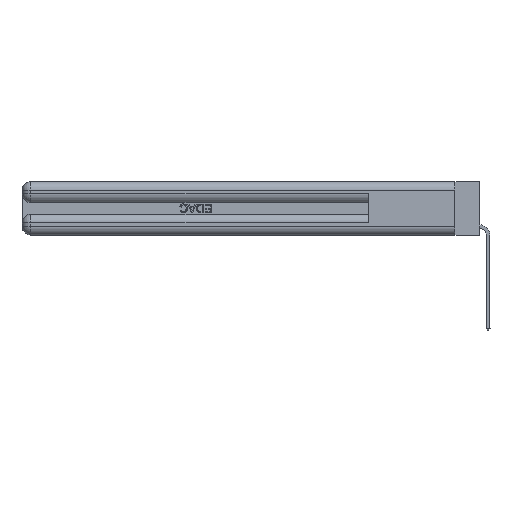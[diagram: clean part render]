
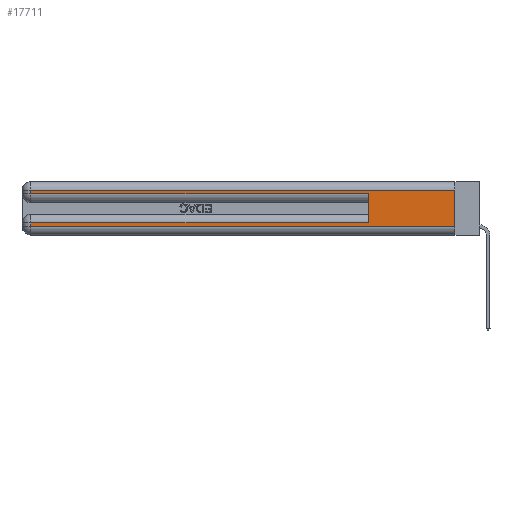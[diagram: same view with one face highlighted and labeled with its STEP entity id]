
A CAD part, left-side view. The second image highlights one B-rep face of the part: STEP entity #17711.
In plain terms, the highlighted planar face has unit normal (-1, 0, 0).
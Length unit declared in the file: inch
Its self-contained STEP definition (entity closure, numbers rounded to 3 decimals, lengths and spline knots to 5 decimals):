
#437 = CARTESIAN_POINT ( 'NONE',  ( 0., 0.6, 0.285 ) ) ;
#541 = AXIS2_PLACEMENT_3D ( 'NONE', #9061, #16422, #13409 ) ;
#1165 = VECTOR ( 'NONE', #8745, 39.37008 ) ;
#1166 = EDGE_CURVE ( 'NONE', #23944, #1646, #4770, .T. ) ;
#1267 = DIRECTION ( 'NONE',  ( 0., 0., -1. ) ) ;
#1416 = EDGE_CURVE ( 'NONE', #3021, #27083, #19693, .T. ) ;
#1646 = VERTEX_POINT ( 'NONE', #437 ) ;
#1948 = EDGE_CURVE ( 'NONE', #26313, #26884, #22142, .T. ) ;
#2638 = VECTOR ( 'NONE', #27305, 39.37008 ) ;
#3021 = VERTEX_POINT ( 'NONE', #27377 ) ;
#3228 = DIRECTION ( 'NONE',  ( 0., 0., -1. ) ) ;
#3637 = ORIENTED_EDGE ( 'NONE', *, *, #15374, .T. ) ;
#3994 = DIRECTION ( 'NONE',  ( 0., 1., 0. ) ) ;
#4770 = LINE ( 'NONE', #9004, #2638 ) ;
#4819 = LINE ( 'NONE', #27820, #1165 ) ;
#6630 = EDGE_CURVE ( 'NONE', #9397, #23944, #10506, .T. ) ;
#6666 = ORIENTED_EDGE ( 'NONE', *, *, #11618, .F. ) ;
#7908 = ORIENTED_EDGE ( 'NONE', *, *, #1948, .T. ) ;
#8669 = CARTESIAN_POINT ( 'NONE',  ( 0., 0., 0.31 ) ) ;
#8745 = DIRECTION ( 'NONE',  ( 0., 1., 0. ) ) ;
#8899 = ORIENTED_EDGE ( 'NONE', *, *, #1416, .F. ) ;
#9004 = CARTESIAN_POINT ( 'NONE',  ( 0., 0., 0.285 ) ) ;
#9061 = CARTESIAN_POINT ( 'NONE',  ( 0., 0., 0.37 ) ) ;
#9397 = VERTEX_POINT ( 'NONE', #14711 ) ;
#10204 = VECTOR ( 'NONE', #1267, 39.37008 ) ;
#10211 = CARTESIAN_POINT ( 'NONE',  ( 0., 2.94, 0.37 ) ) ;
#10324 = LINE ( 'NONE', #12427, #22272 ) ;
#10506 = LINE ( 'NONE', #10211, #10204 ) ;
#10920 = VECTOR ( 'NONE', #24571, 39.37008 ) ;
#11618 = EDGE_CURVE ( 'NONE', #21586, #1646, #10324, .T. ) ;
#12427 = CARTESIAN_POINT ( 'NONE',  ( 0., 0.6, 0.145 ) ) ;
#12752 = CARTESIAN_POINT ( 'NONE',  ( 0., 0., 0.06 ) ) ;
#13189 = LINE ( 'NONE', #8669, #28075 ) ;
#13409 = DIRECTION ( 'NONE',  ( 0., 0., -1. ) ) ;
#13631 = VECTOR ( 'NONE', #23959, 39.37008 ) ;
#13753 = VECTOR ( 'NONE', #3228, 39.37008 ) ;
#14711 = CARTESIAN_POINT ( 'NONE',  ( 0., 2.94, 0.31 ) ) ;
#15320 = CARTESIAN_POINT ( 'NONE',  ( 0., 2.94, 0.37 ) ) ;
#15374 = EDGE_CURVE ( 'NONE', #3021, #9397, #13189, .T. ) ;
#16422 = DIRECTION ( 'NONE',  ( 1., 0., 0. ) ) ;
#17711 = ADVANCED_FACE ( 'NONE', ( #20541 ), #29794, .F. ) ;
#18253 = CARTESIAN_POINT ( 'NONE',  ( 0., 2.94, 0.085 ) ) ;
#19693 = LINE ( 'NONE', #26826, #13753 ) ;
#20541 = FACE_OUTER_BOUND ( 'NONE', #28572, .T. ) ;
#21586 = VERTEX_POINT ( 'NONE', #29789 ) ;
#21800 = CARTESIAN_POINT ( 'NONE',  ( 0., 0., 0.06 ) ) ;
#22142 = LINE ( 'NONE', #15320, #10920 ) ;
#22272 = VECTOR ( 'NONE', #24409, 39.37008 ) ;
#22872 = EDGE_CURVE ( 'NONE', #21586, #26313, #4819, .T. ) ;
#23944 = VERTEX_POINT ( 'NONE', #26923 ) ;
#23959 = DIRECTION ( 'NONE',  ( 0., -1., 0. ) ) ;
#24245 = LINE ( 'NONE', #21800, #13631 ) ;
#24294 = ORIENTED_EDGE ( 'NONE', *, *, #6630, .T. ) ;
#24409 = DIRECTION ( 'NONE',  ( 0., 0., 1. ) ) ;
#24571 = DIRECTION ( 'NONE',  ( 0., 0., -1. ) ) ;
#25219 = CARTESIAN_POINT ( 'NONE',  ( 0., 2.94, 0.06 ) ) ;
#26313 = VERTEX_POINT ( 'NONE', #18253 ) ;
#26826 = CARTESIAN_POINT ( 'NONE',  ( 0., 0., 0.37 ) ) ;
#26884 = VERTEX_POINT ( 'NONE', #25219 ) ;
#26923 = CARTESIAN_POINT ( 'NONE',  ( 0., 2.94, 0.285 ) ) ;
#27083 = VERTEX_POINT ( 'NONE', #12752 ) ;
#27305 = DIRECTION ( 'NONE',  ( 0., -1., 0. ) ) ;
#27377 = CARTESIAN_POINT ( 'NONE',  ( 0., 0., 0.31 ) ) ;
#27820 = CARTESIAN_POINT ( 'NONE',  ( 0., 0., 0.085 ) ) ;
#28075 = VECTOR ( 'NONE', #3994, 39.37008 ) ;
#28439 = ORIENTED_EDGE ( 'NONE', *, *, #1166, .T. ) ;
#28572 = EDGE_LOOP ( 'NONE', ( #8899, #3637, #24294, #28439, #6666, #29715, #7908, #29328 ) ) ;
#29328 = ORIENTED_EDGE ( 'NONE', *, *, #29682, .T. ) ;
#29682 = EDGE_CURVE ( 'NONE', #26884, #27083, #24245, .T. ) ;
#29715 = ORIENTED_EDGE ( 'NONE', *, *, #22872, .T. ) ;
#29789 = CARTESIAN_POINT ( 'NONE',  ( 0., 0.6, 0.085 ) ) ;
#29794 = PLANE ( 'NONE',  #541 ) ;
